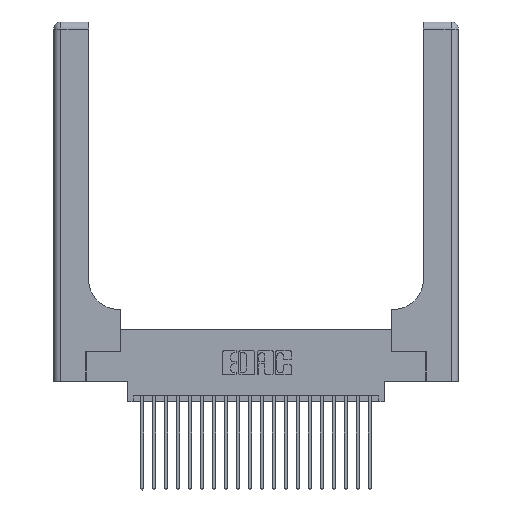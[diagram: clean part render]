
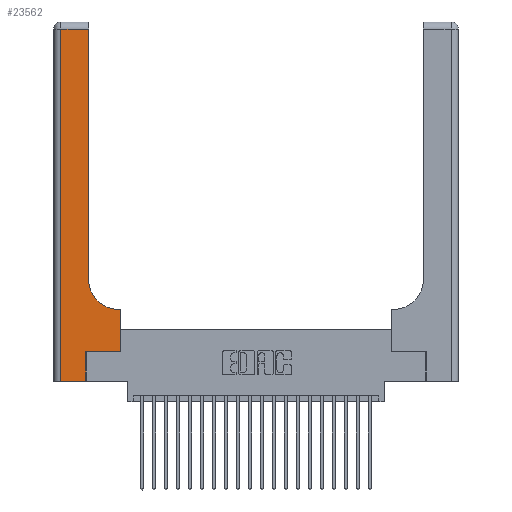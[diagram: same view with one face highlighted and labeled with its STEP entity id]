
A CAD part, top view. The second image highlights one B-rep face of the part: STEP entity #23562.
In plain terms, the highlighted planar face has unit normal (0, 0, 1).
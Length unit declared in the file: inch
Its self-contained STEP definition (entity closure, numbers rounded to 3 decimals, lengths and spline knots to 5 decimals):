
#71 = CARTESIAN_POINT ( 'NONE',  ( 0.5585, 0.25, 0.37 ) ) ;
#196 = CARTESIAN_POINT ( 'NONE',  ( 0.5415, 0.85, 0.37 ) ) ;
#528 = ORIENTED_EDGE ( 'NONE', *, *, #6056, .T. ) ;
#529 = FACE_OUTER_BOUND ( 'NONE', #12436, .T. ) ;
#756 = DIRECTION ( 'NONE',  ( 0., 0., -1. ) ) ;
#1468 = LINE ( 'NONE', #18157, #9294 ) ;
#1889 = CARTESIAN_POINT ( 'NONE',  ( 0.2915, 2.94, 0.37 ) ) ;
#2113 = CARTESIAN_POINT ( 'NONE',  ( 0.2915, 0.6, 0.37 ) ) ;
#2697 = EDGE_CURVE ( 'NONE', #21830, #11735, #8443, .T. ) ;
#2745 = LINE ( 'NONE', #2113, #19283 ) ;
#2755 = LINE ( 'NONE', #6327, #16962 ) ;
#3004 = ORIENTED_EDGE ( 'NONE', *, *, #6785, .T. ) ;
#3506 = VERTEX_POINT ( 'NONE', #4883 ) ;
#3819 = VERTEX_POINT ( 'NONE', #71 ) ;
#4288 = VECTOR ( 'NONE', #7454, 39.37008 ) ;
#4883 = CARTESIAN_POINT ( 'NONE',  ( 0.06, 2.94, 0.37 ) ) ;
#5282 = ORIENTED_EDGE ( 'NONE', *, *, #10014, .T. ) ;
#5576 = CARTESIAN_POINT ( 'NONE',  ( 0.06, 3., 0.37 ) ) ;
#6056 = EDGE_CURVE ( 'NONE', #3819, #12778, #13495, .T. ) ;
#6082 = ORIENTED_EDGE ( 'NONE', *, *, #15074, .T. ) ;
#6327 = CARTESIAN_POINT ( 'NONE',  ( 0.269, 0.25, 0.37 ) ) ;
#6681 = EDGE_CURVE ( 'NONE', #15220, #3819, #2755, .T. ) ;
#6785 = EDGE_CURVE ( 'NONE', #8596, #21428, #8261, .T. ) ;
#7057 = CARTESIAN_POINT ( 'NONE',  ( 0.5415, 0.6, 0.37 ) ) ;
#7394 = CARTESIAN_POINT ( 'NONE',  ( 0.269, 0., 0.37 ) ) ;
#7454 = DIRECTION ( 'NONE',  ( 0., -1., 0. ) ) ;
#8138 = ORIENTED_EDGE ( 'NONE', *, *, #22328, .T. ) ;
#8192 = PLANE ( 'NONE',  #19566 ) ;
#8261 = LINE ( 'NONE', #9122, #10036 ) ;
#8443 = CIRCLE ( 'NONE', #8878, 0.25 ) ;
#8596 = VERTEX_POINT ( 'NONE', #12473 ) ;
#8773 = DIRECTION ( 'NONE',  ( -1., 0., 0. ) ) ;
#8878 = AXIS2_PLACEMENT_3D ( 'NONE', #196, #14847, #22409 ) ;
#9122 = CARTESIAN_POINT ( 'NONE',  ( 0., 0., 0.37 ) ) ;
#9294 = VECTOR ( 'NONE', #8773, 39.37008 ) ;
#9870 = ORIENTED_EDGE ( 'NONE', *, *, #15895, .T. ) ;
#10006 = ORIENTED_EDGE ( 'NONE', *, *, #18062, .T. ) ;
#10014 = EDGE_CURVE ( 'NONE', #18087, #3506, #1468, .T. ) ;
#10036 = VECTOR ( 'NONE', #18425, 39.37008 ) ;
#10306 = DIRECTION ( 'NONE',  ( -1., 0., 0. ) ) ;
#11735 = VERTEX_POINT ( 'NONE', #13702 ) ;
#12390 = LINE ( 'NONE', #5576, #4288 ) ;
#12436 = EDGE_LOOP ( 'NONE', ( #9870, #5282, #6082, #3004, #8138, #22434, #528, #10006, #19150 ) ) ;
#12473 = CARTESIAN_POINT ( 'NONE',  ( 0.06, 0., 0.37 ) ) ;
#12778 = VERTEX_POINT ( 'NONE', #23185 ) ;
#13163 = DIRECTION ( 'NONE',  ( -1., 0., 0. ) ) ;
#13279 = LINE ( 'NONE', #15796, #23201 ) ;
#13495 = LINE ( 'NONE', #13946, #20784 ) ;
#13702 = CARTESIAN_POINT ( 'NONE',  ( 0.2915, 0.85, 0.37 ) ) ;
#13884 = CARTESIAN_POINT ( 'NONE',  ( 0.269, 0., 0.37 ) ) ;
#13920 = DIRECTION ( 'NONE',  ( 0., 1., 0. ) ) ;
#13946 = CARTESIAN_POINT ( 'NONE',  ( 0.5585, 0.25, 0.37 ) ) ;
#14847 = DIRECTION ( 'NONE',  ( 0., 0., -1. ) ) ;
#15053 = LINE ( 'NONE', #13884, #17668 ) ;
#15074 = EDGE_CURVE ( 'NONE', #3506, #8596, #12390, .T. ) ;
#15220 = VERTEX_POINT ( 'NONE', #19407 ) ;
#15796 = CARTESIAN_POINT ( 'NONE',  ( 0.2915, 3., 0.37 ) ) ;
#15895 = EDGE_CURVE ( 'NONE', #11735, #18087, #13279, .T. ) ;
#16325 = DIRECTION ( 'NONE',  ( 0., 1., 0. ) ) ;
#16962 = VECTOR ( 'NONE', #21586, 39.37008 ) ;
#17577 = CARTESIAN_POINT ( 'NONE',  ( 0., 3., 0.37 ) ) ;
#17668 = VECTOR ( 'NONE', #23759, 39.37008 ) ;
#18062 = EDGE_CURVE ( 'NONE', #12778, #21830, #2745, .T. ) ;
#18087 = VERTEX_POINT ( 'NONE', #1889 ) ;
#18157 = CARTESIAN_POINT ( 'NONE',  ( 0., 2.94, 0.37 ) ) ;
#18425 = DIRECTION ( 'NONE',  ( 1., 0., 0. ) ) ;
#19150 = ORIENTED_EDGE ( 'NONE', *, *, #2697, .T. ) ;
#19283 = VECTOR ( 'NONE', #13163, 39.37008 ) ;
#19407 = CARTESIAN_POINT ( 'NONE',  ( 0.269, 0.25, 0.37 ) ) ;
#19566 = AXIS2_PLACEMENT_3D ( 'NONE', #17577, #756, #10306 ) ;
#20784 = VECTOR ( 'NONE', #16325, 39.37008 ) ;
#21428 = VERTEX_POINT ( 'NONE', #7394 ) ;
#21586 = DIRECTION ( 'NONE',  ( 1., 0., 0. ) ) ;
#21830 = VERTEX_POINT ( 'NONE', #7057 ) ;
#22328 = EDGE_CURVE ( 'NONE', #21428, #15220, #15053, .T. ) ;
#22409 = DIRECTION ( 'NONE',  ( 1., 0., 0. ) ) ;
#22434 = ORIENTED_EDGE ( 'NONE', *, *, #6681, .T. ) ;
#23185 = CARTESIAN_POINT ( 'NONE',  ( 0.5585, 0.6, 0.37 ) ) ;
#23201 = VECTOR ( 'NONE', #13920, 39.37008 ) ;
#23562 = ADVANCED_FACE ( 'NONE', ( #529 ), #8192, .F. ) ;
#23759 = DIRECTION ( 'NONE',  ( 0., 1., 0. ) ) ;
